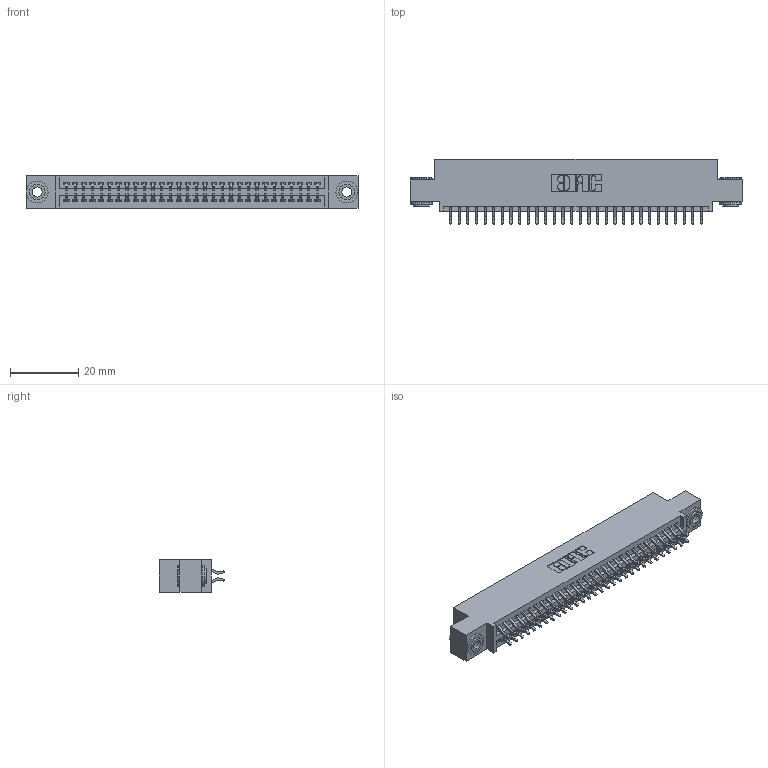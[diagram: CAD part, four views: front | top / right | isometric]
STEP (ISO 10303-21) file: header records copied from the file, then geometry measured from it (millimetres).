
FILE_DESCRIPTION (( 'STEP AP203' ), '1' );
FILE_NAME ('395-060-556-503.STEP', '2019-10-23T14:45:39', ( '' ), ( '' ), 'SwSTEP 2.0', 'SolidWorks 2016', '' );
FILE_SCHEMA (( 'CONFIG_CONTROL_DESIGN' ));
Length unit declared in the file: inch
Products named in the file (4): 345 Part_0.110 Offset - 0.156 Dia-TH; 345-292-001_556 Tail; 345-250-002_345-250-002-102; 395-060-556-503
Assembly tree (63 placements, depth 2):
  395-060-556-503
    345 Part_0.110 Offset - 0.156 Dia-TH
    345-292-001_556 Tail  x60
    345-250-002_345-250-002-102  x2
Bounding box: 97.41 x 19.24 x 9.4 mm (x, y, z)
Volume: 9294.7 mm3; surface area: 13751.9 mm2
Topology: 63 solids, 63 shells, 3528 faces, 10449 edges, 6882 vertices
Faces by surface type: plane 2314, cylinder 1206, cone 8
Entity records: 26156 total; most frequent: CARTESIAN_POINT 4387, ORIENTED_EDGE 4302, DIRECTION 3901, EDGE_CURVE 2151, LINE 1867, VECTOR 1867, VERTEX_POINT 1430, AXIS2_PLACEMENT_3D 1017
